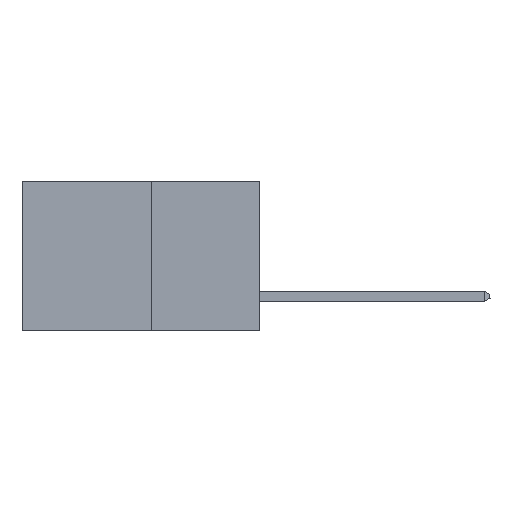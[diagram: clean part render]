
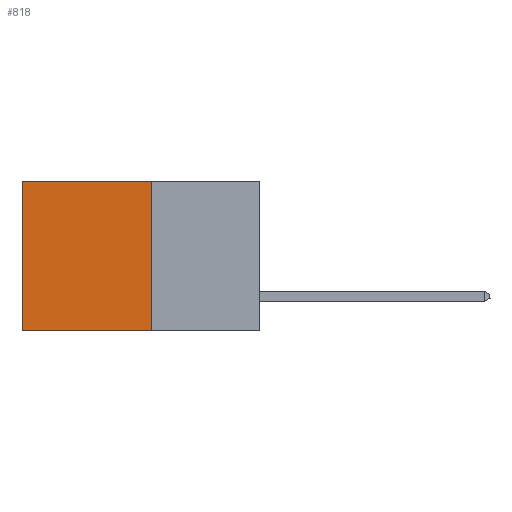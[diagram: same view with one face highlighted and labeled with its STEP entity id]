
A CAD part, left-side view. The second image highlights one B-rep face of the part: STEP entity #818.
In plain terms, the highlighted planar face has unit normal (-1, 0, 0).
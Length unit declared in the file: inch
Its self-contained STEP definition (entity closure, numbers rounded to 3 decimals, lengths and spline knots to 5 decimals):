
#261 = VERTEX_POINT ( 'NONE', #2588 ) ;
#818 = ADVANCED_FACE ( 'NONE', ( #16686 ), #16470, .F. ) ;
#1527 = CARTESIAN_POINT ( 'NONE',  ( 0.277, 0.27, -0.37 ) ) ;
#1553 = DIRECTION ( 'NONE',  ( 0., 1., 0. ) ) ;
#1972 = VERTEX_POINT ( 'NONE', #5644 ) ;
#2588 = CARTESIAN_POINT ( 'NONE',  ( 0.277, 0.27, 0. ) ) ;
#2624 = VECTOR ( 'NONE', #16746, 39.37008 ) ;
#2694 = DIRECTION ( 'NONE',  ( 1., 0., 0. ) ) ;
#2942 = CARTESIAN_POINT ( 'NONE',  ( 0.277, 0.27, -0.37 ) ) ;
#3172 = LINE ( 'NONE', #16823, #2624 ) ;
#3784 = LINE ( 'NONE', #13322, #5719 ) ;
#3802 = EDGE_CURVE ( 'NONE', #12836, #1972, #3172, .T. ) ;
#5540 = VERTEX_POINT ( 'NONE', #2942 ) ;
#5575 = EDGE_CURVE ( 'NONE', #5540, #1972, #21195, .T. ) ;
#5644 = CARTESIAN_POINT ( 'NONE',  ( 0.277, 0.59, -0.37 ) ) ;
#5719 = VECTOR ( 'NONE', #15033, 39.37008 ) ;
#6086 = CARTESIAN_POINT ( 'NONE',  ( 0.277, 0.59, 0. ) ) ;
#7607 = EDGE_LOOP ( 'NONE', ( #8027, #14898, #19939, #15209 ) ) ;
#7799 = DIRECTION ( 'NONE',  ( 0., 0., -1. ) ) ;
#8027 = ORIENTED_EDGE ( 'NONE', *, *, #3802, .T. ) ;
#9527 = EDGE_CURVE ( 'NONE', #261, #5540, #20019, .T. ) ;
#12836 = VERTEX_POINT ( 'NONE', #6086 ) ;
#13322 = CARTESIAN_POINT ( 'NONE',  ( 0.277, 0.27, 0. ) ) ;
#14898 = ORIENTED_EDGE ( 'NONE', *, *, #5575, .F. ) ;
#15033 = DIRECTION ( 'NONE',  ( 0., 1., 0. ) ) ;
#15209 = ORIENTED_EDGE ( 'NONE', *, *, #19914, .T. ) ;
#15545 = VECTOR ( 'NONE', #20052, 39.37008 ) ;
#15551 = AXIS2_PLACEMENT_3D ( 'NONE', #16495, #2694, #7799 ) ;
#16470 = PLANE ( 'NONE',  #15551 ) ;
#16495 = CARTESIAN_POINT ( 'NONE',  ( 0.277, 0.27, -0.37 ) ) ;
#16686 = FACE_OUTER_BOUND ( 'NONE', #7607, .T. ) ;
#16746 = DIRECTION ( 'NONE',  ( 0., 0., -1. ) ) ;
#16823 = CARTESIAN_POINT ( 'NONE',  ( 0.277, 0.59, -0.37 ) ) ;
#16839 = VECTOR ( 'NONE', #1553, 39.37008 ) ;
#19914 = EDGE_CURVE ( 'NONE', #261, #12836, #3784, .T. ) ;
#19939 = ORIENTED_EDGE ( 'NONE', *, *, #9527, .F. ) ;
#20019 = LINE ( 'NONE', #20048, #15545 ) ;
#20048 = CARTESIAN_POINT ( 'NONE',  ( 0.277, 0.27, -0.37 ) ) ;
#20052 = DIRECTION ( 'NONE',  ( 0., 0., -1. ) ) ;
#21195 = LINE ( 'NONE', #1527, #16839 ) ;
